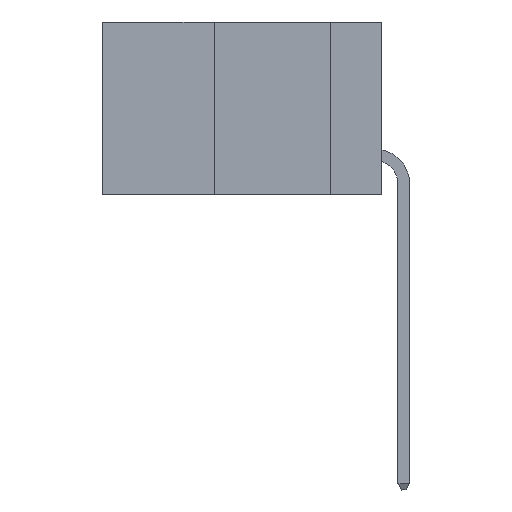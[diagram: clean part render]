
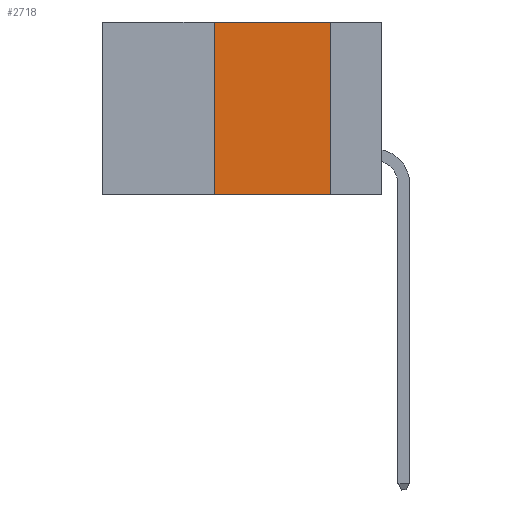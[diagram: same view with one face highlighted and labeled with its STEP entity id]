
A CAD part, left-side view. The second image highlights one B-rep face of the part: STEP entity #2718.
In plain terms, the highlighted planar face has unit normal (-1, 0, 0).
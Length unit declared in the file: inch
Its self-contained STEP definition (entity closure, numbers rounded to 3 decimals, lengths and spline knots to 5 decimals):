
#1429 = PLANE ( 'NONE',  #41902 ) ;
#2267 = EDGE_CURVE ( 'NONE', #18879, #20861, #19167, .T. ) ;
#2718 = ADVANCED_FACE ( 'NONE', ( #31953 ), #1429, .F. ) ;
#4014 = DIRECTION ( 'NONE',  ( 0., 0., -1. ) ) ;
#8674 = DIRECTION ( 'NONE',  ( 0., -1., 0. ) ) ;
#9293 = VECTOR ( 'NONE', #4014, 39.37008 ) ;
#9473 = EDGE_CURVE ( 'NONE', #22129, #18879, #20318, .T. ) ;
#10796 = LINE ( 'NONE', #20780, #9293 ) ;
#12116 = CARTESIAN_POINT ( 'NONE',  ( 0., 0.6, 0. ) ) ;
#12348 = VECTOR ( 'NONE', #31828, 39.37008 ) ;
#12795 = EDGE_CURVE ( 'NONE', #20861, #14638, #10796, .T. ) ;
#13287 = VECTOR ( 'NONE', #15377, 39.37008 ) ;
#14638 = VERTEX_POINT ( 'NONE', #21963 ) ;
#15377 = DIRECTION ( 'NONE',  ( 0., -1., 0. ) ) ;
#15655 = CARTESIAN_POINT ( 'NONE',  ( 0., 0.6, 0. ) ) ;
#18879 = VERTEX_POINT ( 'NONE', #37554 ) ;
#19162 = CARTESIAN_POINT ( 'NONE',  ( 0., 0.6, -0.37 ) ) ;
#19167 = LINE ( 'NONE', #12116, #13287 ) ;
#20318 = LINE ( 'NONE', #29163, #12348 ) ;
#20780 = CARTESIAN_POINT ( 'NONE',  ( 0., 0.11, 0. ) ) ;
#20861 = VERTEX_POINT ( 'NONE', #21908 ) ;
#20974 = CARTESIAN_POINT ( 'NONE',  ( 0., 0.36, -0.37 ) ) ;
#21908 = CARTESIAN_POINT ( 'NONE',  ( 0., 0.11, 0. ) ) ;
#21963 = CARTESIAN_POINT ( 'NONE',  ( 0., 0.11, -0.37 ) ) ;
#22129 = VERTEX_POINT ( 'NONE', #20974 ) ;
#22651 = DIRECTION ( 'NONE',  ( 0., 0., -1. ) ) ;
#25311 = ORIENTED_EDGE ( 'NONE', *, *, #9473, .F. ) ;
#29163 = CARTESIAN_POINT ( 'NONE',  ( 0., 0.36, 0. ) ) ;
#30583 = EDGE_CURVE ( 'NONE', #22129, #14638, #31746, .T. ) ;
#31147 = EDGE_LOOP ( 'NONE', ( #36878, #42117, #25311, #40206 ) ) ;
#31746 = LINE ( 'NONE', #19162, #35486 ) ;
#31828 = DIRECTION ( 'NONE',  ( 0., 0., 1. ) ) ;
#31953 = FACE_OUTER_BOUND ( 'NONE', #31147, .T. ) ;
#35486 = VECTOR ( 'NONE', #8674, 39.37008 ) ;
#36878 = ORIENTED_EDGE ( 'NONE', *, *, #12795, .F. ) ;
#37554 = CARTESIAN_POINT ( 'NONE',  ( 0., 0.36, 0. ) ) ;
#39668 = DIRECTION ( 'NONE',  ( 1., 0., 0. ) ) ;
#40206 = ORIENTED_EDGE ( 'NONE', *, *, #30583, .T. ) ;
#41902 = AXIS2_PLACEMENT_3D ( 'NONE', #15655, #39668, #22651 ) ;
#42117 = ORIENTED_EDGE ( 'NONE', *, *, #2267, .F. ) ;
